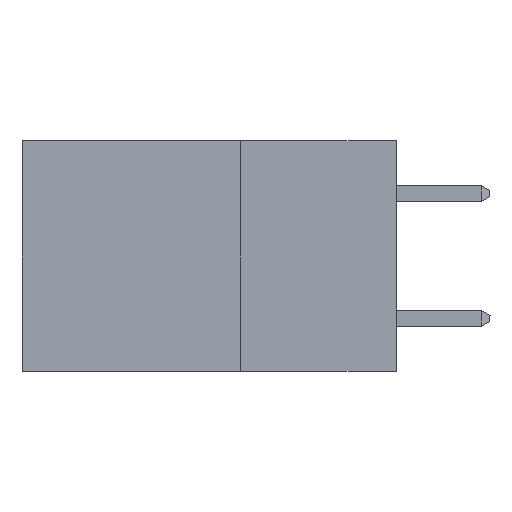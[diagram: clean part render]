
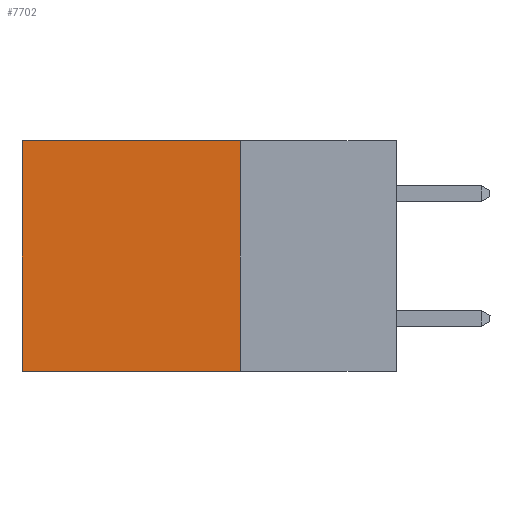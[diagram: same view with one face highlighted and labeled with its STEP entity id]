
A CAD part, left-side view. The second image highlights one B-rep face of the part: STEP entity #7702.
In plain terms, the highlighted planar face has unit normal (-1, 0, 0).
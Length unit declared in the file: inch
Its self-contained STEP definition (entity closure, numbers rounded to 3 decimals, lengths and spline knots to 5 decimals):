
#1071 = DIRECTION ( 'NONE',  ( 0., 1., 0. ) ) ;
#1117 = ORIENTED_EDGE ( 'NONE', *, *, #6987, .F. ) ;
#1222 = EDGE_LOOP ( 'NONE', ( #8719, #1117, #8271, #4926 ) ) ;
#1549 = EDGE_CURVE ( 'NONE', #16444, #10257, #2372, .T. ) ;
#1579 = CARTESIAN_POINT ( 'NONE',  ( 0.2615, 0.25, -0.37 ) ) ;
#1984 = FACE_OUTER_BOUND ( 'NONE', #1222, .T. ) ;
#2111 = EDGE_CURVE ( 'NONE', #13535, #9893, #11124, .T. ) ;
#2372 = LINE ( 'NONE', #12261, #18657 ) ;
#3261 = VECTOR ( 'NONE', #19661, 39.37008 ) ;
#4926 = ORIENTED_EDGE ( 'NONE', *, *, #19082, .T. ) ;
#6950 = CARTESIAN_POINT ( 'NONE',  ( 0.2615, 0.6, -0.37 ) ) ;
#6987 = EDGE_CURVE ( 'NONE', #9893, #10257, #11289, .T. ) ;
#7702 = ADVANCED_FACE ( 'NONE', ( #1984 ), #18894, .F. ) ;
#8271 = ORIENTED_EDGE ( 'NONE', *, *, #2111, .F. ) ;
#8719 = ORIENTED_EDGE ( 'NONE', *, *, #1549, .T. ) ;
#9264 = CARTESIAN_POINT ( 'NONE',  ( 0.2615, 0.25, -0.37 ) ) ;
#9893 = VERTEX_POINT ( 'NONE', #9264 ) ;
#10119 = VECTOR ( 'NONE', #15151, 39.37008 ) ;
#10257 = VERTEX_POINT ( 'NONE', #6950 ) ;
#10670 = CARTESIAN_POINT ( 'NONE',  ( 0.2615, 0.25, 0. ) ) ;
#11124 = LINE ( 'NONE', #1579, #10119 ) ;
#11172 = VECTOR ( 'NONE', #1071, 39.37008 ) ;
#11289 = LINE ( 'NONE', #19747, #3261 ) ;
#12261 = CARTESIAN_POINT ( 'NONE',  ( 0.2615, 0.6, -0.37 ) ) ;
#13535 = VERTEX_POINT ( 'NONE', #18724 ) ;
#15151 = DIRECTION ( 'NONE',  ( 0., 0., -1. ) ) ;
#16444 = VERTEX_POINT ( 'NONE', #18680 ) ;
#17657 = AXIS2_PLACEMENT_3D ( 'NONE', #18666, #18530, #18516 ) ;
#18516 = DIRECTION ( 'NONE',  ( 0., 0., -1. ) ) ;
#18530 = DIRECTION ( 'NONE',  ( 1., 0., 0. ) ) ;
#18657 = VECTOR ( 'NONE', #18901, 39.37008 ) ;
#18666 = CARTESIAN_POINT ( 'NONE',  ( 0.2615, 0.25, -0.37 ) ) ;
#18680 = CARTESIAN_POINT ( 'NONE',  ( 0.2615, 0.6, 0. ) ) ;
#18724 = CARTESIAN_POINT ( 'NONE',  ( 0.2615, 0.25, 0. ) ) ;
#18894 = PLANE ( 'NONE',  #17657 ) ;
#18901 = DIRECTION ( 'NONE',  ( 0., 0., -1. ) ) ;
#19082 = EDGE_CURVE ( 'NONE', #13535, #16444, #19385, .T. ) ;
#19385 = LINE ( 'NONE', #10670, #11172 ) ;
#19661 = DIRECTION ( 'NONE',  ( 0., 1., 0. ) ) ;
#19747 = CARTESIAN_POINT ( 'NONE',  ( 0.2615, 0.25, -0.37 ) ) ;
